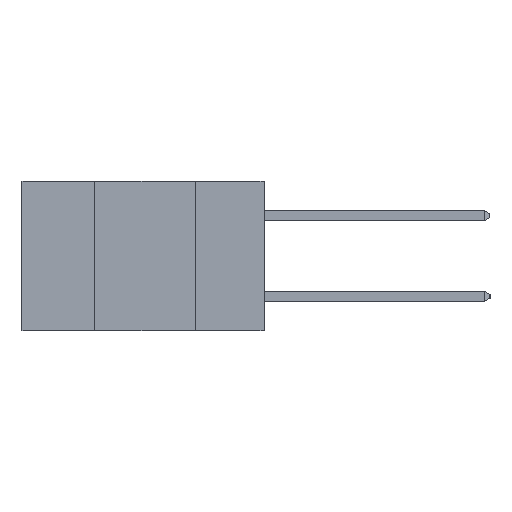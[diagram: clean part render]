
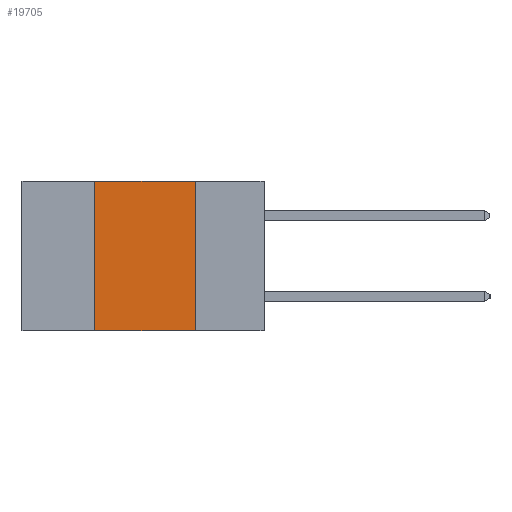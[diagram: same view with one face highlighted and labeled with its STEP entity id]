
A CAD part, left-side view. The second image highlights one B-rep face of the part: STEP entity #19705.
In plain terms, the highlighted planar face has unit normal (-1, 0, 0).
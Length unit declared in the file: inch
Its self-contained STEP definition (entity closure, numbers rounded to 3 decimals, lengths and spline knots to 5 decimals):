
#3303 = ORIENTED_EDGE ( 'NONE', *, *, #17578, .T. ) ;
#3787 = DIRECTION ( 'NONE',  ( 0., -1., 0. ) ) ;
#4340 = LINE ( 'NONE', #7052, #18599 ) ;
#5733 = AXIS2_PLACEMENT_3D ( 'NONE', #15423, #17187, #6496 ) ;
#6496 = DIRECTION ( 'NONE',  ( 0., 0., -1. ) ) ;
#6650 = CARTESIAN_POINT ( 'NONE',  ( 0., 0.17, -0.37 ) ) ;
#6832 = CARTESIAN_POINT ( 'NONE',  ( 0., 0.42, 0. ) ) ;
#7052 = CARTESIAN_POINT ( 'NONE',  ( 0., 0.42, -0.37 ) ) ;
#7610 = EDGE_CURVE ( 'NONE', #22363, #9152, #23179, .T. ) ;
#8874 = DIRECTION ( 'NONE',  ( 0., 0., 1. ) ) ;
#9152 = VERTEX_POINT ( 'NONE', #17005 ) ;
#9868 = VECTOR ( 'NONE', #22800, 39.37008 ) ;
#9929 = VERTEX_POINT ( 'NONE', #13121 ) ;
#11669 = EDGE_CURVE ( 'NONE', #9152, #16637, #19260, .T. ) ;
#13121 = CARTESIAN_POINT ( 'NONE',  ( 0., 0.42, -0.37 ) ) ;
#13130 = CARTESIAN_POINT ( 'NONE',  ( 0., 0.6, 0. ) ) ;
#13529 = VECTOR ( 'NONE', #3787, 39.37008 ) ;
#13652 = PLANE ( 'NONE',  #5733 ) ;
#13688 = FACE_OUTER_BOUND ( 'NONE', #20766, .T. ) ;
#13856 = VECTOR ( 'NONE', #14909, 39.37008 ) ;
#14909 = DIRECTION ( 'NONE',  ( 0., -1., 0. ) ) ;
#15423 = CARTESIAN_POINT ( 'NONE',  ( 0., 0.6, 0. ) ) ;
#16637 = VERTEX_POINT ( 'NONE', #6650 ) ;
#16955 = ORIENTED_EDGE ( 'NONE', *, *, #11669, .F. ) ;
#17005 = CARTESIAN_POINT ( 'NONE',  ( 0., 0.17, 0. ) ) ;
#17187 = DIRECTION ( 'NONE',  ( 1., 0., 0. ) ) ;
#17578 = EDGE_CURVE ( 'NONE', #9929, #16637, #21221, .T. ) ;
#18050 = CARTESIAN_POINT ( 'NONE',  ( 0., 0.6, -0.37 ) ) ;
#18599 = VECTOR ( 'NONE', #8874, 39.37008 ) ;
#19260 = LINE ( 'NONE', #21045, #9868 ) ;
#19705 = ADVANCED_FACE ( 'NONE', ( #13688 ), #13652, .F. ) ;
#19925 = EDGE_CURVE ( 'NONE', #9929, #22363, #4340, .T. ) ;
#20766 = EDGE_LOOP ( 'NONE', ( #16955, #21660, #21658, #3303 ) ) ;
#21045 = CARTESIAN_POINT ( 'NONE',  ( 0., 0.17, -0.37 ) ) ;
#21221 = LINE ( 'NONE', #18050, #13529 ) ;
#21658 = ORIENTED_EDGE ( 'NONE', *, *, #19925, .F. ) ;
#21660 = ORIENTED_EDGE ( 'NONE', *, *, #7610, .F. ) ;
#22363 = VERTEX_POINT ( 'NONE', #6832 ) ;
#22800 = DIRECTION ( 'NONE',  ( 0., 0., -1. ) ) ;
#23179 = LINE ( 'NONE', #13130, #13856 ) ;
